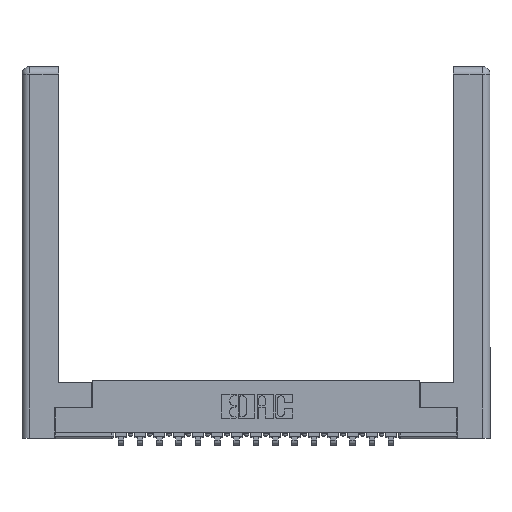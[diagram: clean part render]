
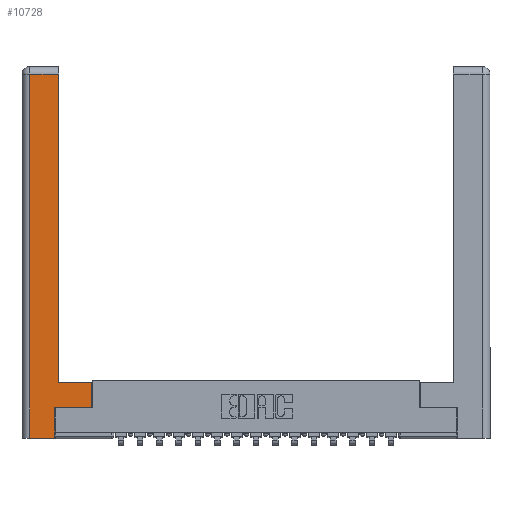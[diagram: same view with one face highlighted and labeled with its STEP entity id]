
A CAD part, top view. The second image highlights one B-rep face of the part: STEP entity #10728.
In plain terms, the highlighted planar face has unit normal (0, 0, 1).
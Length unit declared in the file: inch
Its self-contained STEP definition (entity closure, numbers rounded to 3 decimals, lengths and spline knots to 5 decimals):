
#122 = CARTESIAN_POINT ( 'NONE',  ( 0.265, 0.245, 0. ) ) ;
#346 = EDGE_CURVE ( 'NONE', #17296, #10428, #3304, .T. ) ;
#623 = LINE ( 'NONE', #12869, #9106 ) ;
#802 = CARTESIAN_POINT ( 'NONE',  ( 0.0615, 0., 0. ) ) ;
#1195 = VECTOR ( 'NONE', #1715, 39.37008 ) ;
#1404 = CARTESIAN_POINT ( 'NONE',  ( 0.0615, 0., 0. ) ) ;
#1715 = DIRECTION ( 'NONE',  ( -1., 0., 0. ) ) ;
#1807 = EDGE_CURVE ( 'NONE', #4498, #18064, #6643, .T. ) ;
#2303 = DIRECTION ( 'NONE',  ( 0., 1., 0. ) ) ;
#2451 = VERTEX_POINT ( 'NONE', #5526 ) ;
#2671 = ORIENTED_EDGE ( 'NONE', *, *, #346, .T. ) ;
#2782 = CARTESIAN_POINT ( 'NONE',  ( 0.295, 0.45, 0. ) ) ;
#2860 = VECTOR ( 'NONE', #16137, 39.37008 ) ;
#2978 = VERTEX_POINT ( 'NONE', #14944 ) ;
#3304 = LINE ( 'NONE', #9755, #13387 ) ;
#4039 = EDGE_CURVE ( 'NONE', #2451, #2978, #623, .T. ) ;
#4402 = ORIENTED_EDGE ( 'NONE', *, *, #9347, .T. ) ;
#4498 = VERTEX_POINT ( 'NONE', #802 ) ;
#4701 = CARTESIAN_POINT ( 'NONE',  ( 0.565, 0.245, 0. ) ) ;
#5388 = VERTEX_POINT ( 'NONE', #18804 ) ;
#5526 = CARTESIAN_POINT ( 'NONE',  ( 0.295, 0.45, 0. ) ) ;
#6076 = EDGE_CURVE ( 'NONE', #2978, #5388, #16646, .T. ) ;
#6188 = CARTESIAN_POINT ( 'NONE',  ( 0.0615, 2.94, 0. ) ) ;
#6643 = LINE ( 'NONE', #17195, #15382 ) ;
#7435 = DIRECTION ( 'NONE',  ( -1., 0., 0. ) ) ;
#8243 = LINE ( 'NONE', #17010, #19480 ) ;
#8436 = VERTEX_POINT ( 'NONE', #12803 ) ;
#8785 = DIRECTION ( 'NONE',  ( -1., 0., 0. ) ) ;
#9095 = ORIENTED_EDGE ( 'NONE', *, *, #4039, .T. ) ;
#9101 = ORIENTED_EDGE ( 'NONE', *, *, #19267, .T. ) ;
#9106 = VECTOR ( 'NONE', #11282, 39.37008 ) ;
#9347 = EDGE_CURVE ( 'NONE', #18064, #17296, #11155, .T. ) ;
#9556 = CARTESIAN_POINT ( 'NONE',  ( 0.265, 0.245, 0. ) ) ;
#9755 = CARTESIAN_POINT ( 'NONE',  ( 0.565, 0.245, 0. ) ) ;
#9831 = DIRECTION ( 'NONE',  ( 0., 1., 0. ) ) ;
#10048 = CARTESIAN_POINT ( 'NONE',  ( 0.265, 0., 0. ) ) ;
#10160 = PLANE ( 'NONE',  #18831 ) ;
#10264 = CARTESIAN_POINT ( 'NONE',  ( 0., 0., 0. ) ) ;
#10428 = VERTEX_POINT ( 'NONE', #4701 ) ;
#10728 = ADVANCED_FACE ( 'NONE', ( #13148 ), #10160, .F. ) ;
#11063 = EDGE_CURVE ( 'NONE', #10428, #8436, #8243, .T. ) ;
#11155 = LINE ( 'NONE', #9556, #18757 ) ;
#11282 = DIRECTION ( 'NONE',  ( 0., 1., 0. ) ) ;
#11592 = ORIENTED_EDGE ( 'NONE', *, *, #1807, .T. ) ;
#12803 = CARTESIAN_POINT ( 'NONE',  ( 0.565, 0.45, 0. ) ) ;
#12869 = CARTESIAN_POINT ( 'NONE',  ( 0.295, 3., 0. ) ) ;
#13079 = ORIENTED_EDGE ( 'NONE', *, *, #11063, .T. ) ;
#13134 = ORIENTED_EDGE ( 'NONE', *, *, #6076, .T. ) ;
#13148 = FACE_OUTER_BOUND ( 'NONE', #14484, .T. ) ;
#13387 = VECTOR ( 'NONE', #15751, 39.37008 ) ;
#14484 = EDGE_LOOP ( 'NONE', ( #9095, #13134, #9101, #11592, #4402, #2671, #13079, #18043 ) ) ;
#14748 = DIRECTION ( 'NONE',  ( 0., 0., -1. ) ) ;
#14944 = CARTESIAN_POINT ( 'NONE',  ( 0.295, 2.94, 0. ) ) ;
#15382 = VECTOR ( 'NONE', #15816, 39.37008 ) ;
#15751 = DIRECTION ( 'NONE',  ( 1., 0., 0. ) ) ;
#15816 = DIRECTION ( 'NONE',  ( 1., 0., 0. ) ) ;
#16137 = DIRECTION ( 'NONE',  ( 0., -1., 0. ) ) ;
#16470 = EDGE_CURVE ( 'NONE', #8436, #2451, #19397, .T. ) ;
#16534 = LINE ( 'NONE', #1404, #2860 ) ;
#16646 = LINE ( 'NONE', #6188, #1195 ) ;
#17010 = CARTESIAN_POINT ( 'NONE',  ( 0.565, 0.45, 0. ) ) ;
#17195 = CARTESIAN_POINT ( 'NONE',  ( 0.265, 0., 0. ) ) ;
#17296 = VERTEX_POINT ( 'NONE', #122 ) ;
#17698 = VECTOR ( 'NONE', #7435, 39.37008 ) ;
#18043 = ORIENTED_EDGE ( 'NONE', *, *, #16470, .T. ) ;
#18064 = VERTEX_POINT ( 'NONE', #10048 ) ;
#18757 = VECTOR ( 'NONE', #2303, 39.37008 ) ;
#18804 = CARTESIAN_POINT ( 'NONE',  ( 0.0615, 2.94, 0. ) ) ;
#18831 = AXIS2_PLACEMENT_3D ( 'NONE', #10264, #14748, #8785 ) ;
#19267 = EDGE_CURVE ( 'NONE', #5388, #4498, #16534, .T. ) ;
#19397 = LINE ( 'NONE', #2782, #17698 ) ;
#19480 = VECTOR ( 'NONE', #9831, 39.37008 ) ;
